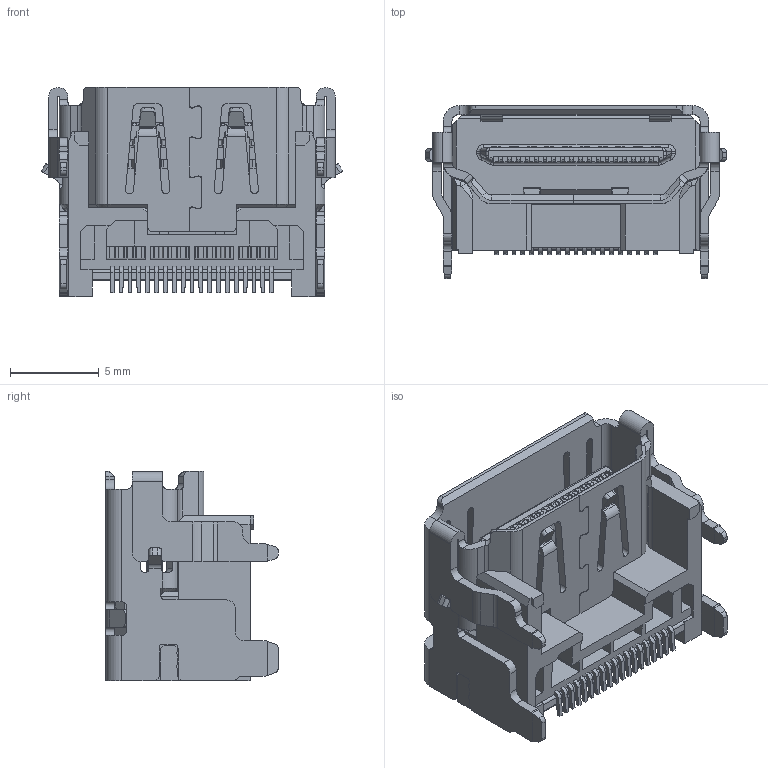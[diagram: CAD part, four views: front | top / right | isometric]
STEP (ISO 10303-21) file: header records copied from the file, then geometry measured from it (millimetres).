
FILE_DESCRIPTION (( 'STEP AP214' ), '1' );
FILE_NAME ('694D119-163-111.STEP', '2021-01-13T16:22:59', ( '' ), ( '' ), 'SwSTEP 2.0', 'SolidWorks 2020', '' );
FILE_SCHEMA (( 'AUTOMOTIVE_DESIGN' ));
Length unit declared in the file: millimetre
Products named in the file (4): Contacts 694D119-X63-111; Insulator 694D119-X63-111; 694D119-163-111; Shell 694D119-X63-111
Assembly tree (3 placements, depth 2):
  694D119-163-111
    Insulator 694D119-X63-111
    Contacts 694D119-X63-111
    Shell 694D119-X63-111
Bounding box: 17.01 x 9.75 x 11.8 mm (x, y, z)
Volume: 548.9 mm3; surface area: 2209.7 mm2
Topology: 21 solids, 21 shells, 3479 faces, 9855 edges, 6384 vertices
Faces by surface type: plane 2261, cylinder 1100, bspline 56, sphere 52, cone 10
Entity records: 114400 total; most frequent: CARTESIAN_POINT 22662, ORIENTED_EDGE 19702, DIRECTION 18542, EDGE_CURVE 9851, LINE 7496, VECTOR 7496, VERTEX_POINT 6384, AXIS2_PLACEMENT_3D 5523
